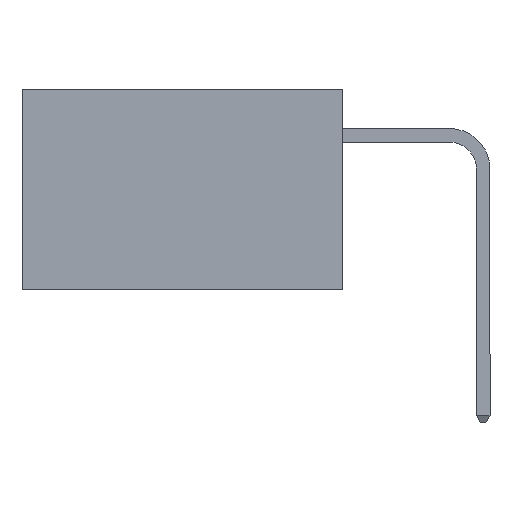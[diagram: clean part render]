
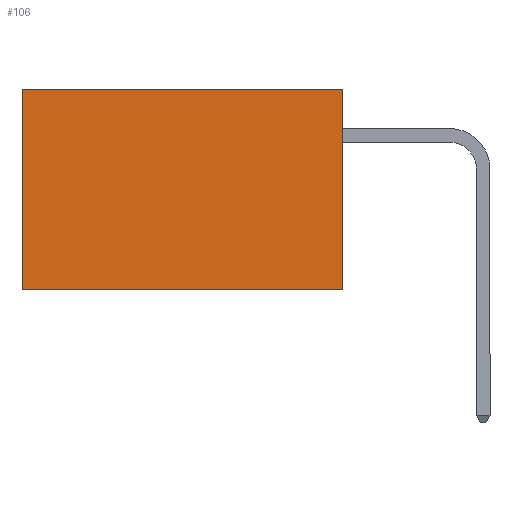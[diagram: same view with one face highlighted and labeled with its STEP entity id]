
A CAD part, left-side view. The second image highlights one B-rep face of the part: STEP entity #106.
In plain terms, the highlighted planar face has unit normal (-1, 0, 0).
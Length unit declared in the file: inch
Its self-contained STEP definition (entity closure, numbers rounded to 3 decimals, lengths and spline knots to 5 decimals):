
#106 = ADVANCED_FACE ( 'NONE', ( #851 ), #2065, .F. ) ;
#228 = VERTEX_POINT ( 'NONE', #6681 ) ;
#851 = FACE_OUTER_BOUND ( 'NONE', #6925, .T. ) ;
#1202 = VERTEX_POINT ( 'NONE', #8087 ) ;
#1965 = DIRECTION ( 'NONE',  ( 0., 0., -1. ) ) ;
#2065 = PLANE ( 'NONE',  #5704 ) ;
#2238 = CARTESIAN_POINT ( 'NONE',  ( 0.277, 0., 0. ) ) ;
#2268 = DIRECTION ( 'NONE',  ( 0., 1., 0. ) ) ;
#2410 = VERTEX_POINT ( 'NONE', #5668 ) ;
#2515 = VECTOR ( 'NONE', #4655, 39.37008 ) ;
#2984 = LINE ( 'NONE', #4762, #4689 ) ;
#4282 = VECTOR ( 'NONE', #2268, 39.37008 ) ;
#4506 = LINE ( 'NONE', #2238, #4282 ) ;
#4567 = CARTESIAN_POINT ( 'NONE',  ( 0.277, 0.59, -0.37 ) ) ;
#4655 = DIRECTION ( 'NONE',  ( 0., 0., -1. ) ) ;
#4689 = VECTOR ( 'NONE', #4973, 39.37008 ) ;
#4762 = CARTESIAN_POINT ( 'NONE',  ( 0.277, 0., -0.37 ) ) ;
#4973 = DIRECTION ( 'NONE',  ( 0., 1., 0. ) ) ;
#5198 = CARTESIAN_POINT ( 'NONE',  ( 0.277, 0.59, -0.37 ) ) ;
#5286 = DIRECTION ( 'NONE',  ( 0., 0., -1. ) ) ;
#5453 = CARTESIAN_POINT ( 'NONE',  ( 0.277, 0., -0.37 ) ) ;
#5580 = CARTESIAN_POINT ( 'NONE',  ( 0.277, 0., -0.37 ) ) ;
#5668 = CARTESIAN_POINT ( 'NONE',  ( 0.277, 0.59, 0. ) ) ;
#5704 = AXIS2_PLACEMENT_3D ( 'NONE', #5453, #7248, #1965 ) ;
#5750 = EDGE_CURVE ( 'NONE', #1202, #228, #8026, .T. ) ;
#6132 = VECTOR ( 'NONE', #5286, 39.37008 ) ;
#6307 = VERTEX_POINT ( 'NONE', #5198 ) ;
#6681 = CARTESIAN_POINT ( 'NONE',  ( 0.277, 0., -0.37 ) ) ;
#6925 = EDGE_LOOP ( 'NONE', ( #7227, #7444, #7963, #8378 ) ) ;
#7227 = ORIENTED_EDGE ( 'NONE', *, *, #7382, .T. ) ;
#7248 = DIRECTION ( 'NONE',  ( 1., 0., 0. ) ) ;
#7324 = EDGE_CURVE ( 'NONE', #228, #6307, #2984, .T. ) ;
#7382 = EDGE_CURVE ( 'NONE', #2410, #6307, #8436, .T. ) ;
#7444 = ORIENTED_EDGE ( 'NONE', *, *, #7324, .F. ) ;
#7963 = ORIENTED_EDGE ( 'NONE', *, *, #5750, .F. ) ;
#8026 = LINE ( 'NONE', #5580, #6132 ) ;
#8087 = CARTESIAN_POINT ( 'NONE',  ( 0.277, 0., 0. ) ) ;
#8378 = ORIENTED_EDGE ( 'NONE', *, *, #9371, .T. ) ;
#8436 = LINE ( 'NONE', #4567, #2515 ) ;
#9371 = EDGE_CURVE ( 'NONE', #1202, #2410, #4506, .T. ) ;
